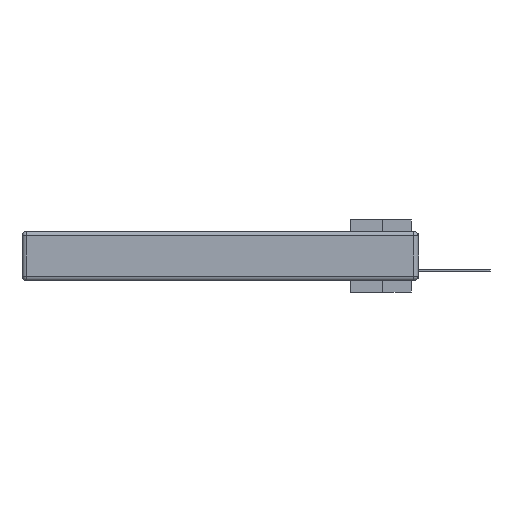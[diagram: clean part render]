
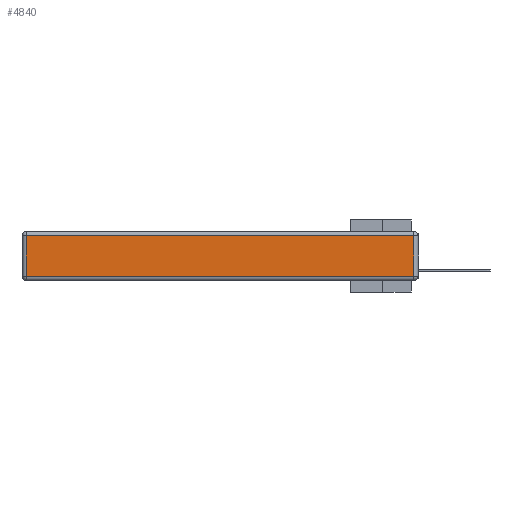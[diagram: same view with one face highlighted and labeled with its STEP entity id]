
A CAD part, left-side view. The second image highlights one B-rep face of the part: STEP entity #4840.
In plain terms, the highlighted planar face has unit normal (-1, 0, 0).
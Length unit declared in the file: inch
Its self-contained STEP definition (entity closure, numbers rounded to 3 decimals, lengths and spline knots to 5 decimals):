
#836 = CARTESIAN_POINT ( 'NONE',  ( 0., 2.75, -0.03 ) ) ;
#970 = VECTOR ( 'NONE', #13701, 39.37008 ) ;
#1675 = LINE ( 'NONE', #15520, #26195 ) ;
#1876 = VECTOR ( 'NONE', #19781, 39.37008 ) ;
#4224 = CARTESIAN_POINT ( 'NONE',  ( 0., 0.03, -0.343 ) ) ;
#4355 = EDGE_CURVE ( 'NONE', #23315, #18405, #10169, .T. ) ;
#4840 = ADVANCED_FACE ( 'NONE', ( #18489 ), #20658, .T. ) ;
#4948 = LINE ( 'NONE', #24038, #20528 ) ;
#5311 = EDGE_CURVE ( 'NONE', #17329, #26658, #1675, .T. ) ;
#7335 = ORIENTED_EDGE ( 'NONE', *, *, #28955, .T. ) ;
#7652 = CARTESIAN_POINT ( 'NONE',  ( 0., 0.03, -0.03 ) ) ;
#7965 = EDGE_CURVE ( 'NONE', #26658, #23315, #25475, .T. ) ;
#10169 = LINE ( 'NONE', #836, #1876 ) ;
#13701 = DIRECTION ( 'NONE',  ( 0., 0., 1. ) ) ;
#14840 = CARTESIAN_POINT ( 'NONE',  ( 0., 2.72, -0.313 ) ) ;
#15333 = ORIENTED_EDGE ( 'NONE', *, *, #4355, .T. ) ;
#15520 = CARTESIAN_POINT ( 'NONE',  ( 0., 0., -0.313 ) ) ;
#15788 = AXIS2_PLACEMENT_3D ( 'NONE', #18187, #30114, #29663 ) ;
#17329 = VERTEX_POINT ( 'NONE', #14840 ) ;
#18187 = CARTESIAN_POINT ( 'NONE',  ( 0., 0., -0.343 ) ) ;
#18405 = VERTEX_POINT ( 'NONE', #23201 ) ;
#18489 = FACE_OUTER_BOUND ( 'NONE', #21561, .T. ) ;
#19781 = DIRECTION ( 'NONE',  ( 0., 1., 0. ) ) ;
#20316 = DIRECTION ( 'NONE',  ( 0., -1., 0. ) ) ;
#20528 = VECTOR ( 'NONE', #23881, 39.37008 ) ;
#20658 = PLANE ( 'NONE',  #15788 ) ;
#21561 = EDGE_LOOP ( 'NONE', ( #24729, #22880, #15333, #7335 ) ) ;
#22516 = CARTESIAN_POINT ( 'NONE',  ( 0., 0.03, -0.313 ) ) ;
#22880 = ORIENTED_EDGE ( 'NONE', *, *, #7965, .T. ) ;
#23201 = CARTESIAN_POINT ( 'NONE',  ( 0., 2.72, -0.03 ) ) ;
#23315 = VERTEX_POINT ( 'NONE', #7652 ) ;
#23881 = DIRECTION ( 'NONE',  ( 0., 0., -1. ) ) ;
#24038 = CARTESIAN_POINT ( 'NONE',  ( 0., 2.72, -0.343 ) ) ;
#24729 = ORIENTED_EDGE ( 'NONE', *, *, #5311, .T. ) ;
#25475 = LINE ( 'NONE', #4224, #970 ) ;
#26195 = VECTOR ( 'NONE', #20316, 39.37008 ) ;
#26658 = VERTEX_POINT ( 'NONE', #22516 ) ;
#28955 = EDGE_CURVE ( 'NONE', #18405, #17329, #4948, .T. ) ;
#29663 = DIRECTION ( 'NONE',  ( 0., 0., 1. ) ) ;
#30114 = DIRECTION ( 'NONE',  ( -1., 0., 0. ) ) ;
